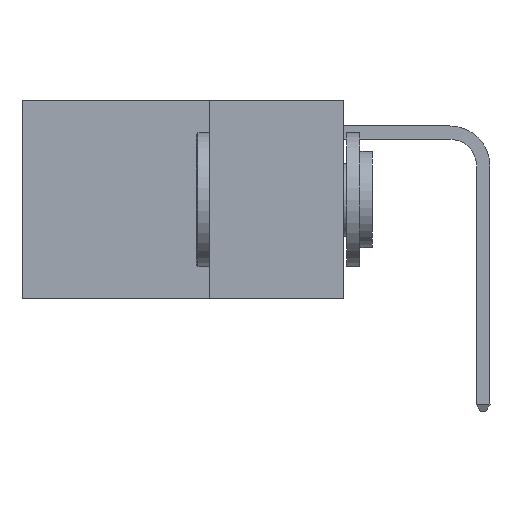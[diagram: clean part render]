
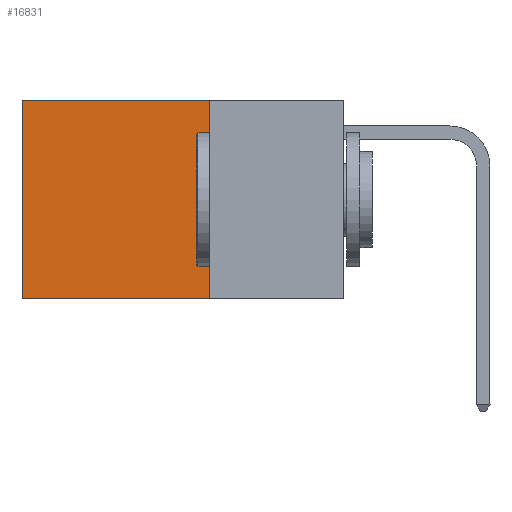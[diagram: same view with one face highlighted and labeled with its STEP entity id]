
A CAD part, left-side view. The second image highlights one B-rep face of the part: STEP entity #16831.
In plain terms, the highlighted planar face has unit normal (-1, 0, 0).
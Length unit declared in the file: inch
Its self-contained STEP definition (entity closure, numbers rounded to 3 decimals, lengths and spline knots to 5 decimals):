
#150 = DIRECTION ( 'NONE',  ( 0., 0., -1. ) ) ;
#403 = ORIENTED_EDGE ( 'NONE', *, *, #19389, .F. ) ;
#815 = ORIENTED_EDGE ( 'NONE', *, *, #12087, .T. ) ;
#1703 = VECTOR ( 'NONE', #11154, 39.37008 ) ;
#1874 = VERTEX_POINT ( 'NONE', #5228 ) ;
#2120 = LINE ( 'NONE', #10953, #12159 ) ;
#3288 = CARTESIAN_POINT ( 'NONE',  ( 0.2625, 0.25, 0. ) ) ;
#5228 = CARTESIAN_POINT ( 'NONE',  ( 0.2625, 0.25, -0.37 ) ) ;
#7169 = LINE ( 'NONE', #20045, #8894 ) ;
#7224 = DIRECTION ( 'NONE',  ( 0., 0., -1. ) ) ;
#7449 = VERTEX_POINT ( 'NONE', #9146 ) ;
#7546 = DIRECTION ( 'NONE',  ( 0., 1., 0. ) ) ;
#7784 = VERTEX_POINT ( 'NONE', #11836 ) ;
#8894 = VECTOR ( 'NONE', #14820, 39.37008 ) ;
#9146 = CARTESIAN_POINT ( 'NONE',  ( 0.2625, 0.6, 0. ) ) ;
#10311 = VECTOR ( 'NONE', #150, 39.37008 ) ;
#10953 = CARTESIAN_POINT ( 'NONE',  ( 0.2625, 0.25, 0. ) ) ;
#11154 = DIRECTION ( 'NONE',  ( 0., 0., -1. ) ) ;
#11836 = CARTESIAN_POINT ( 'NONE',  ( 0.2625, 0.6, -0.37 ) ) ;
#12087 = EDGE_CURVE ( 'NONE', #7449, #7784, #19806, .T. ) ;
#12159 = VECTOR ( 'NONE', #7546, 39.37008 ) ;
#12637 = PLANE ( 'NONE',  #15444 ) ;
#12982 = ORIENTED_EDGE ( 'NONE', *, *, #13441, .F. ) ;
#13207 = VERTEX_POINT ( 'NONE', #3288 ) ;
#13441 = EDGE_CURVE ( 'NONE', #1874, #7784, #7169, .T. ) ;
#14668 = LINE ( 'NONE', #20110, #10311 ) ;
#14820 = DIRECTION ( 'NONE',  ( 0., 1., 0. ) ) ;
#15386 = ORIENTED_EDGE ( 'NONE', *, *, #18694, .T. ) ;
#15444 = AXIS2_PLACEMENT_3D ( 'NONE', #17861, #19640, #7224 ) ;
#15862 = FACE_OUTER_BOUND ( 'NONE', #21301, .T. ) ;
#16831 = ADVANCED_FACE ( 'NONE', ( #15862 ), #12637, .F. ) ;
#17861 = CARTESIAN_POINT ( 'NONE',  ( 0.2625, 0.25, 0. ) ) ;
#18694 = EDGE_CURVE ( 'NONE', #13207, #7449, #2120, .T. ) ;
#19389 = EDGE_CURVE ( 'NONE', #13207, #1874, #14668, .T. ) ;
#19640 = DIRECTION ( 'NONE',  ( 1., 0., 0. ) ) ;
#19691 = CARTESIAN_POINT ( 'NONE',  ( 0.2625, 0.6, 0. ) ) ;
#19806 = LINE ( 'NONE', #19691, #1703 ) ;
#20045 = CARTESIAN_POINT ( 'NONE',  ( 0.2625, 0.25, -0.37 ) ) ;
#20110 = CARTESIAN_POINT ( 'NONE',  ( 0.2625, 0.25, 0. ) ) ;
#21301 = EDGE_LOOP ( 'NONE', ( #815, #12982, #403, #15386 ) ) ;
